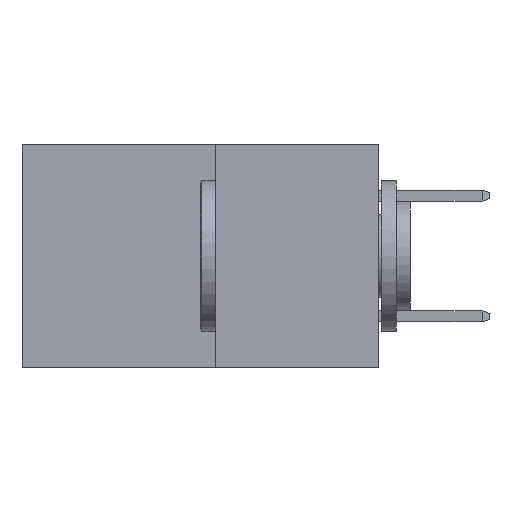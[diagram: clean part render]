
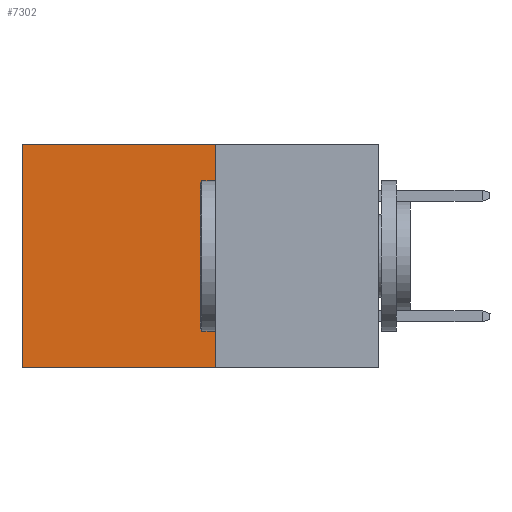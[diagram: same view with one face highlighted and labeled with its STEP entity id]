
A CAD part, left-side view. The second image highlights one B-rep face of the part: STEP entity #7302.
In plain terms, the highlighted planar face has unit normal (-1, 0, 0).
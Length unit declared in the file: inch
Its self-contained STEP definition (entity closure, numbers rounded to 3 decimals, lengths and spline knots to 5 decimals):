
#695 = EDGE_CURVE ( 'NONE', #3745, #8280, #3561, .T. ) ;
#938 = ORIENTED_EDGE ( 'NONE', *, *, #2185, .F. ) ;
#1119 = CARTESIAN_POINT ( 'NONE',  ( 0.277, 0.59, 0. ) ) ;
#1789 = VERTEX_POINT ( 'NONE', #6013 ) ;
#1814 = ORIENTED_EDGE ( 'NONE', *, *, #695, .T. ) ;
#1891 = EDGE_CURVE ( 'NONE', #1789, #3745, #10800, .T. ) ;
#1977 = DIRECTION ( 'NONE',  ( 0., 0., -1. ) ) ;
#2185 = EDGE_CURVE ( 'NONE', #1789, #10074, #4980, .T. ) ;
#2744 = EDGE_LOOP ( 'NONE', ( #1814, #8663, #938, #4552 ) ) ;
#2940 = DIRECTION ( 'NONE',  ( 0., 1., 0. ) ) ;
#3561 = LINE ( 'NONE', #10930, #7750 ) ;
#3630 = CARTESIAN_POINT ( 'NONE',  ( 0.277, 0.27, -0.37 ) ) ;
#3664 = CARTESIAN_POINT ( 'NONE',  ( 0.277, 0.27, -0.37 ) ) ;
#3745 = VERTEX_POINT ( 'NONE', #1119 ) ;
#4081 = EDGE_CURVE ( 'NONE', #10074, #8280, #8712, .T. ) ;
#4552 = ORIENTED_EDGE ( 'NONE', *, *, #1891, .T. ) ;
#4637 = DIRECTION ( 'NONE',  ( 0., 1., 0. ) ) ;
#4980 = LINE ( 'NONE', #10883, #8894 ) ;
#4999 = CARTESIAN_POINT ( 'NONE',  ( 0.277, 0.59, -0.37 ) ) ;
#5543 = CARTESIAN_POINT ( 'NONE',  ( 0.277, 0.27, -0.37 ) ) ;
#5743 = CARTESIAN_POINT ( 'NONE',  ( 0.277, 0.27, 0. ) ) ;
#6013 = CARTESIAN_POINT ( 'NONE',  ( 0.277, 0.27, 0. ) ) ;
#6659 = VECTOR ( 'NONE', #4637, 39.37008 ) ;
#7301 = DIRECTION ( 'NONE',  ( 1., 0., 0. ) ) ;
#7302 = ADVANCED_FACE ( 'NONE', ( #9409 ), #9585, .F. ) ;
#7750 = VECTOR ( 'NONE', #8648, 39.37008 ) ;
#8280 = VERTEX_POINT ( 'NONE', #4999 ) ;
#8648 = DIRECTION ( 'NONE',  ( 0., 0., -1. ) ) ;
#8663 = ORIENTED_EDGE ( 'NONE', *, *, #4081, .F. ) ;
#8712 = LINE ( 'NONE', #3664, #6659 ) ;
#8764 = VECTOR ( 'NONE', #2940, 39.37008 ) ;
#8894 = VECTOR ( 'NONE', #10773, 39.37008 ) ;
#9409 = FACE_OUTER_BOUND ( 'NONE', #2744, .T. ) ;
#9585 = PLANE ( 'NONE',  #10241 ) ;
#10074 = VERTEX_POINT ( 'NONE', #3630 ) ;
#10241 = AXIS2_PLACEMENT_3D ( 'NONE', #5543, #7301, #1977 ) ;
#10773 = DIRECTION ( 'NONE',  ( 0., 0., -1. ) ) ;
#10800 = LINE ( 'NONE', #5743, #8764 ) ;
#10883 = CARTESIAN_POINT ( 'NONE',  ( 0.277, 0.27, -0.37 ) ) ;
#10930 = CARTESIAN_POINT ( 'NONE',  ( 0.277, 0.59, -0.37 ) ) ;
